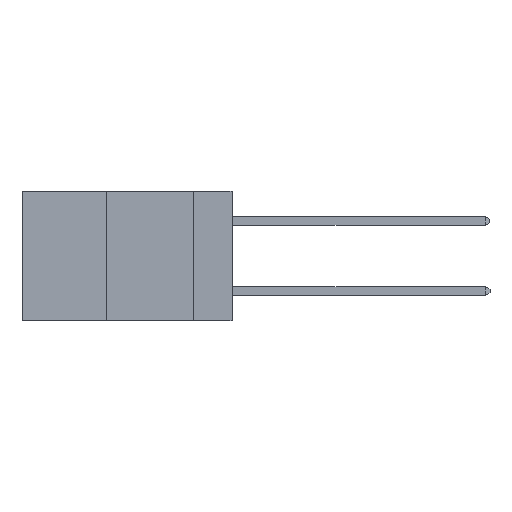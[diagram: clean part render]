
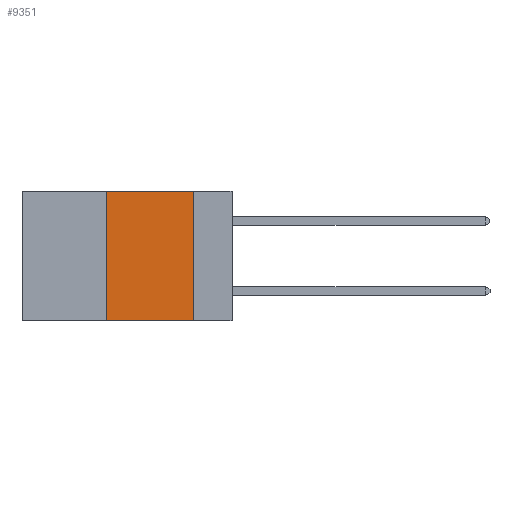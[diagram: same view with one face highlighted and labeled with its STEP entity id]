
A CAD part, left-side view. The second image highlights one B-rep face of the part: STEP entity #9351.
In plain terms, the highlighted planar face has unit normal (-1, 0, 0).
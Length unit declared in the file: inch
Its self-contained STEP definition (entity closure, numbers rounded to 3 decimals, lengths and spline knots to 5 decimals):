
#32 = LINE ( 'NONE', #16683, #7312 ) ;
#201 = DIRECTION ( 'NONE',  ( 1., 0., 0. ) ) ;
#385 = CARTESIAN_POINT ( 'NONE',  ( 0., 0.6, 0. ) ) ;
#1712 = VERTEX_POINT ( 'NONE', #5423 ) ;
#1839 = CARTESIAN_POINT ( 'NONE',  ( 0., 0.11, 0. ) ) ;
#2793 = ORIENTED_EDGE ( 'NONE', *, *, #6503, .F. ) ;
#2808 = ORIENTED_EDGE ( 'NONE', *, *, #14472, .F. ) ;
#4018 = CARTESIAN_POINT ( 'NONE',  ( 0., 0.36, 0. ) ) ;
#4410 = ORIENTED_EDGE ( 'NONE', *, *, #8738, .T. ) ;
#5036 = EDGE_CURVE ( 'NONE', #5228, #1712, #5929, .T. ) ;
#5228 = VERTEX_POINT ( 'NONE', #1839 ) ;
#5423 = CARTESIAN_POINT ( 'NONE',  ( 0., 0.11, -0.37 ) ) ;
#5726 = CARTESIAN_POINT ( 'NONE',  ( 0., 0.6, -0.37 ) ) ;
#5929 = LINE ( 'NONE', #9591, #16008 ) ;
#5973 = FACE_OUTER_BOUND ( 'NONE', #9611, .T. ) ;
#6133 = DIRECTION ( 'NONE',  ( 0., 0., 1. ) ) ;
#6503 = EDGE_CURVE ( 'NONE', #15715, #12023, #32, .T. ) ;
#6686 = ORIENTED_EDGE ( 'NONE', *, *, #5036, .F. ) ;
#7017 = PLANE ( 'NONE',  #8728 ) ;
#7029 = DIRECTION ( 'NONE',  ( 0., -1., 0. ) ) ;
#7312 = VECTOR ( 'NONE', #6133, 39.37008 ) ;
#7986 = VECTOR ( 'NONE', #15138, 39.37008 ) ;
#8491 = LINE ( 'NONE', #5726, #15072 ) ;
#8728 = AXIS2_PLACEMENT_3D ( 'NONE', #16240, #201, #9747 ) ;
#8738 = EDGE_CURVE ( 'NONE', #15715, #1712, #8491, .T. ) ;
#9351 = ADVANCED_FACE ( 'NONE', ( #5973 ), #7017, .F. ) ;
#9591 = CARTESIAN_POINT ( 'NONE',  ( 0., 0.11, 0. ) ) ;
#9611 = EDGE_LOOP ( 'NONE', ( #6686, #2808, #2793, #4410 ) ) ;
#9747 = DIRECTION ( 'NONE',  ( 0., 0., -1. ) ) ;
#12023 = VERTEX_POINT ( 'NONE', #4018 ) ;
#14472 = EDGE_CURVE ( 'NONE', #12023, #5228, #15404, .T. ) ;
#15072 = VECTOR ( 'NONE', #7029, 39.37008 ) ;
#15138 = DIRECTION ( 'NONE',  ( 0., -1., 0. ) ) ;
#15404 = LINE ( 'NONE', #385, #7986 ) ;
#15715 = VERTEX_POINT ( 'NONE', #16963 ) ;
#16008 = VECTOR ( 'NONE', #16129, 39.37008 ) ;
#16129 = DIRECTION ( 'NONE',  ( 0., 0., -1. ) ) ;
#16240 = CARTESIAN_POINT ( 'NONE',  ( 0., 0.6, 0. ) ) ;
#16683 = CARTESIAN_POINT ( 'NONE',  ( 0., 0.36, 0. ) ) ;
#16963 = CARTESIAN_POINT ( 'NONE',  ( 0., 0.36, -0.37 ) ) ;
